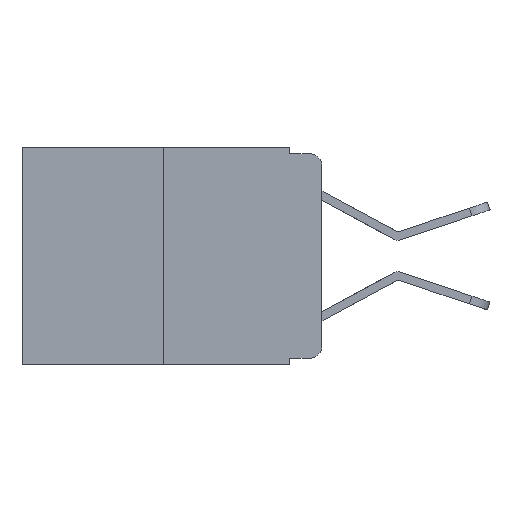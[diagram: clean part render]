
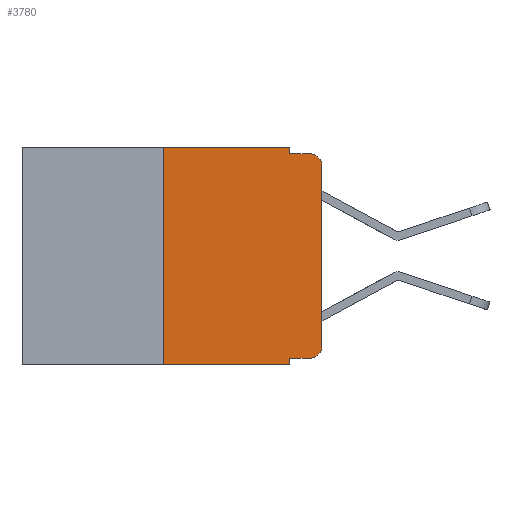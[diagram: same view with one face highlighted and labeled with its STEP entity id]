
A CAD part, left-side view. The second image highlights one B-rep face of the part: STEP entity #3780.
In plain terms, the highlighted planar face has unit normal (-1, 0, 0).
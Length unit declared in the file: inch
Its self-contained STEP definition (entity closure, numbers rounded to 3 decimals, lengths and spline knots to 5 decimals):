
#144 = ORIENTED_EDGE ( 'NONE', *, *, #6341, .T. ) ;
#219 = ORIENTED_EDGE ( 'NONE', *, *, #16091, .T. ) ;
#459 = VECTOR ( 'NONE', #16773, 39.37008 ) ;
#541 = ORIENTED_EDGE ( 'NONE', *, *, #15783, .F. ) ;
#676 = LINE ( 'NONE', #15018, #8151 ) ;
#711 = PLANE ( 'NONE',  #10689 ) ;
#749 = VECTOR ( 'NONE', #1654, 39.37008 ) ;
#968 = VECTOR ( 'NONE', #5651, 39.37008 ) ;
#1035 = EDGE_CURVE ( 'NONE', #11125, #8852, #13032, .T. ) ;
#1389 = LINE ( 'NONE', #15075, #749 ) ;
#1431 = DIRECTION ( 'NONE',  ( -1., 0., 0. ) ) ;
#1654 = DIRECTION ( 'NONE',  ( 0., -1., 0. ) ) ;
#1908 = CARTESIAN_POINT ( 'NONE',  ( 0., 0.473, 0. ) ) ;
#1928 = CARTESIAN_POINT ( 'NONE',  ( 0., 0.051, -0.333 ) ) ;
#2160 = DIRECTION ( 'NONE',  ( 0., 0., 1. ) ) ;
#2325 = ORIENTED_EDGE ( 'NONE', *, *, #11879, .F. ) ;
#2443 = ORIENTED_EDGE ( 'NONE', *, *, #12980, .T. ) ;
#2786 = VERTEX_POINT ( 'NONE', #10510 ) ;
#2916 = VECTOR ( 'NONE', #2160, 39.37008 ) ;
#3059 = AXIS2_PLACEMENT_3D ( 'NONE', #9594, #1431, #11055 ) ;
#3775 = CARTESIAN_POINT ( 'NONE',  ( 0., 0.02, -0.333 ) ) ;
#3780 = ADVANCED_FACE ( 'NONE', ( #11324 ), #711, .F. ) ;
#3808 = CARTESIAN_POINT ( 'NONE',  ( 0., 0.02, -0.03 ) ) ;
#4604 = EDGE_CURVE ( 'NONE', #9148, #11125, #676, .T. ) ;
#4694 = DIRECTION ( 'NONE',  ( 0., 0., -1. ) ) ;
#5135 = CARTESIAN_POINT ( 'NONE',  ( 0., 0.25, -0.343 ) ) ;
#5651 = DIRECTION ( 'NONE',  ( 0., 0., 1. ) ) ;
#5666 = ORIENTED_EDGE ( 'NONE', *, *, #1035, .F. ) ;
#5978 = CIRCLE ( 'NONE', #3059, 0.02 ) ;
#6062 = CARTESIAN_POINT ( 'NONE',  ( 0., 0.051, -0.01 ) ) ;
#6111 = DIRECTION ( 'NONE',  ( 0., -1., 0. ) ) ;
#6262 = DIRECTION ( 'NONE',  ( 0., 0., -1. ) ) ;
#6341 = EDGE_CURVE ( 'NONE', #10638, #17290, #15938, .T. ) ;
#6453 = DIRECTION ( 'NONE',  ( 0., 0., -1. ) ) ;
#6760 = EDGE_CURVE ( 'NONE', #2786, #9148, #13975, .T. ) ;
#7002 = VECTOR ( 'NONE', #15433, 39.37008 ) ;
#7715 = CIRCLE ( 'NONE', #11941, 0.02 ) ;
#7819 = DIRECTION ( 'NONE',  ( -1., 0., 0. ) ) ;
#8151 = VECTOR ( 'NONE', #16397, 39.37008 ) ;
#8278 = ORIENTED_EDGE ( 'NONE', *, *, #12955, .T. ) ;
#8386 = CARTESIAN_POINT ( 'NONE',  ( 0., 0., 0. ) ) ;
#8852 = VERTEX_POINT ( 'NONE', #16844 ) ;
#9148 = VERTEX_POINT ( 'NONE', #14649 ) ;
#9498 = VERTEX_POINT ( 'NONE', #5135 ) ;
#9594 = CARTESIAN_POINT ( 'NONE',  ( 0., 0.02, -0.313 ) ) ;
#10262 = CARTESIAN_POINT ( 'NONE',  ( 0., 0.25, 0. ) ) ;
#10417 = ORIENTED_EDGE ( 'NONE', *, *, #4604, .F. ) ;
#10510 = CARTESIAN_POINT ( 'NONE',  ( 0., 0.25, 0. ) ) ;
#10638 = VERTEX_POINT ( 'NONE', #17111 ) ;
#10689 = AXIS2_PLACEMENT_3D ( 'NONE', #14250, #12961, #6262 ) ;
#10790 = VERTEX_POINT ( 'NONE', #16165 ) ;
#11055 = DIRECTION ( 'NONE',  ( 0., 0., -1. ) ) ;
#11125 = VERTEX_POINT ( 'NONE', #6062 ) ;
#11324 = FACE_OUTER_BOUND ( 'NONE', #11591, .T. ) ;
#11591 = EDGE_LOOP ( 'NONE', ( #8278, #12222, #5666, #10417, #16328, #2325, #2443, #541, #144, #219 ) ) ;
#11772 = CARTESIAN_POINT ( 'NONE',  ( 0., 0.051, 0. ) ) ;
#11877 = VECTOR ( 'NONE', #6111, 39.37008 ) ;
#11879 = EDGE_CURVE ( 'NONE', #9498, #2786, #16120, .T. ) ;
#11941 = AXIS2_PLACEMENT_3D ( 'NONE', #3808, #7819, #6453 ) ;
#12222 = ORIENTED_EDGE ( 'NONE', *, *, #15698, .T. ) ;
#12955 = EDGE_CURVE ( 'NONE', #15656, #10790, #16694, .T. ) ;
#12961 = DIRECTION ( 'NONE',  ( 1., 0., 0. ) ) ;
#12980 = EDGE_CURVE ( 'NONE', #9498, #15602, #1389, .T. ) ;
#13032 = LINE ( 'NONE', #15517, #459 ) ;
#13154 = CARTESIAN_POINT ( 'NONE',  ( 0., 0., -0.313 ) ) ;
#13644 = VECTOR ( 'NONE', #4694, 39.37008 ) ;
#13975 = LINE ( 'NONE', #1908, #7002 ) ;
#14250 = CARTESIAN_POINT ( 'NONE',  ( 0., 0.473, 0. ) ) ;
#14487 = LINE ( 'NONE', #11772, #13644 ) ;
#14649 = CARTESIAN_POINT ( 'NONE',  ( 0., 0.051, 0. ) ) ;
#15018 = CARTESIAN_POINT ( 'NONE',  ( 0., 0.051, 0. ) ) ;
#15075 = CARTESIAN_POINT ( 'NONE',  ( 0., 0.473, -0.343 ) ) ;
#15396 = CARTESIAN_POINT ( 'NONE',  ( 0., 0.051, -0.343 ) ) ;
#15433 = DIRECTION ( 'NONE',  ( 0., -1., 0. ) ) ;
#15517 = CARTESIAN_POINT ( 'NONE',  ( 0., 0.051, -0.01 ) ) ;
#15602 = VERTEX_POINT ( 'NONE', #15396 ) ;
#15656 = VERTEX_POINT ( 'NONE', #13154 ) ;
#15698 = EDGE_CURVE ( 'NONE', #10790, #8852, #7715, .T. ) ;
#15783 = EDGE_CURVE ( 'NONE', #10638, #15602, #14487, .T. ) ;
#15938 = LINE ( 'NONE', #1928, #11877 ) ;
#16091 = EDGE_CURVE ( 'NONE', #17290, #15656, #5978, .T. ) ;
#16120 = LINE ( 'NONE', #10262, #2916 ) ;
#16165 = CARTESIAN_POINT ( 'NONE',  ( 0., 0., -0.03 ) ) ;
#16328 = ORIENTED_EDGE ( 'NONE', *, *, #6760, .F. ) ;
#16397 = DIRECTION ( 'NONE',  ( 0., 0., -1. ) ) ;
#16694 = LINE ( 'NONE', #8386, #968 ) ;
#16773 = DIRECTION ( 'NONE',  ( 0., -1., 0. ) ) ;
#16844 = CARTESIAN_POINT ( 'NONE',  ( 0., 0.02, -0.01 ) ) ;
#17111 = CARTESIAN_POINT ( 'NONE',  ( 0., 0.051, -0.333 ) ) ;
#17290 = VERTEX_POINT ( 'NONE', #3775 ) ;
